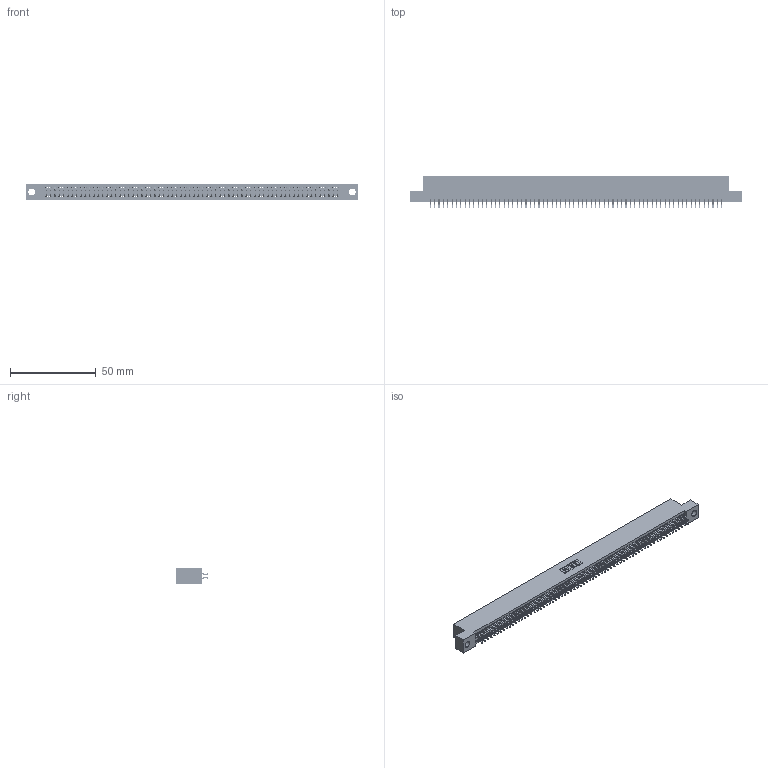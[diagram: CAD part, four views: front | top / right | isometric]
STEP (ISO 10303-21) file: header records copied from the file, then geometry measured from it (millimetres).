
FILE_DESCRIPTION (( 'STEP AP203' ), '1' );
FILE_NAME ('395-136-556-204.STEP', '2018-12-05T10:31:56', ( '' ), ( '' ), 'SwSTEP 2.0', 'SolidWorks 2016', '' );
FILE_SCHEMA (( 'CONFIG_CONTROL_DESIGN' ));
Length unit declared in the file: inch
Products named in the file (3): 395-136-556-204; 345 Part_Flush Mounting Lugs - 0.156 Dia-TH; 345-292-001_556 Tail
Assembly tree (137 placements, depth 2):
  395-136-556-204
    345 Part_Flush Mounting Lugs - 0.156 Dia-TH
    345-292-001_556 Tail  x136
Bounding box: 193.93 x 19.24 x 9.4 mm (x, y, z)
Volume: 18986.6 mm3; surface area: 28265 mm2
Topology: 137 solids, 137 shells, 7742 faces, 23053 edges, 15186 vertices
Faces by surface type: plane 5112, cylinder 2630
Entity records: 50077 total; most frequent: CARTESIAN_POINT 8384, ORIENTED_EDGE 8306, DIRECTION 7349, EDGE_CURVE 4153, LINE 3741, VECTOR 3741, VERTEX_POINT 2766, AXIS2_PLACEMENT_3D 1804
